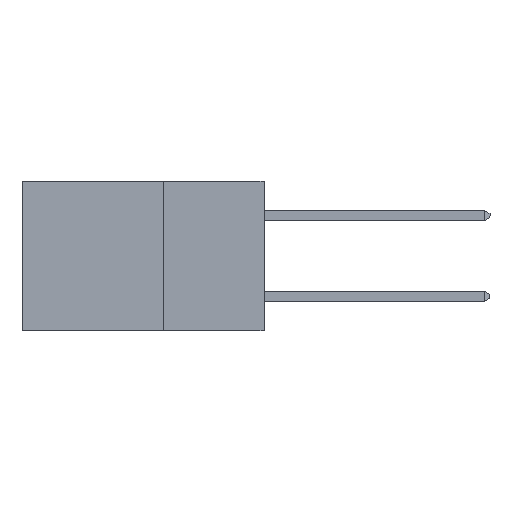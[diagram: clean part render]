
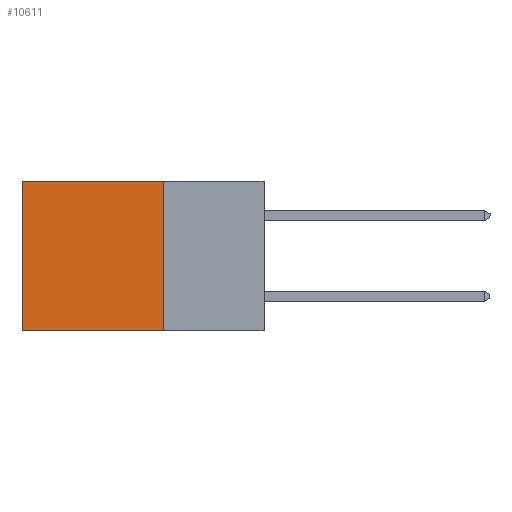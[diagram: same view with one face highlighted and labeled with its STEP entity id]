
A CAD part, left-side view. The second image highlights one B-rep face of the part: STEP entity #10611.
In plain terms, the highlighted planar face has unit normal (-1, 0, 0).
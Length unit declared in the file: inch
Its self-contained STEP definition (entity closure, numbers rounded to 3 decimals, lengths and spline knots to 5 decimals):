
#682 = ORIENTED_EDGE ( 'NONE', *, *, #5136, .F. ) ;
#966 = DIRECTION ( 'NONE',  ( 0., 1., 0. ) ) ;
#1851 = VERTEX_POINT ( 'NONE', #8330 ) ;
#2114 = LINE ( 'NONE', #11177, #6764 ) ;
#2707 = ORIENTED_EDGE ( 'NONE', *, *, #10987, .F. ) ;
#3085 = CARTESIAN_POINT ( 'NONE',  ( 0.298, 0.25, 0. ) ) ;
#3201 = VERTEX_POINT ( 'NONE', #9493 ) ;
#3386 = DIRECTION ( 'NONE',  ( 1., 0., 0. ) ) ;
#3942 = VECTOR ( 'NONE', #6633, 39.37008 ) ;
#4386 = EDGE_LOOP ( 'NONE', ( #4885, #682, #2707, #10275 ) ) ;
#4885 = ORIENTED_EDGE ( 'NONE', *, *, #10183, .T. ) ;
#5136 = EDGE_CURVE ( 'NONE', #7282, #1851, #2114, .T. ) ;
#5416 = CARTESIAN_POINT ( 'NONE',  ( 0.298, 0.6, 0. ) ) ;
#6179 = DIRECTION ( 'NONE',  ( 0., 1., 0. ) ) ;
#6264 = DIRECTION ( 'NONE',  ( 0., 0., -1. ) ) ;
#6286 = LINE ( 'NONE', #3085, #3942 ) ;
#6452 = CARTESIAN_POINT ( 'NONE',  ( 0.298, 0.25, -0.37 ) ) ;
#6633 = DIRECTION ( 'NONE',  ( 0., 0., -1. ) ) ;
#6764 = VECTOR ( 'NONE', #6179, 39.37008 ) ;
#7086 = EDGE_CURVE ( 'NONE', #9172, #3201, #10523, .T. ) ;
#7282 = VERTEX_POINT ( 'NONE', #6452 ) ;
#7370 = VECTOR ( 'NONE', #6264, 39.37008 ) ;
#7472 = LINE ( 'NONE', #5416, #7370 ) ;
#8310 = FACE_OUTER_BOUND ( 'NONE', #4386, .T. ) ;
#8330 = CARTESIAN_POINT ( 'NONE',  ( 0.298, 0.6, -0.37 ) ) ;
#8332 = VECTOR ( 'NONE', #966, 39.37008 ) ;
#8426 = AXIS2_PLACEMENT_3D ( 'NONE', #8607, #3386, #9435 ) ;
#8607 = CARTESIAN_POINT ( 'NONE',  ( 0.298, 0.25, 0. ) ) ;
#8758 = CARTESIAN_POINT ( 'NONE',  ( 0.298, 0.25, 0. ) ) ;
#9141 = CARTESIAN_POINT ( 'NONE',  ( 0.298, 0.25, 0. ) ) ;
#9172 = VERTEX_POINT ( 'NONE', #9141 ) ;
#9435 = DIRECTION ( 'NONE',  ( 0., 0., -1. ) ) ;
#9493 = CARTESIAN_POINT ( 'NONE',  ( 0.298, 0.6, 0. ) ) ;
#10183 = EDGE_CURVE ( 'NONE', #3201, #1851, #7472, .T. ) ;
#10275 = ORIENTED_EDGE ( 'NONE', *, *, #7086, .T. ) ;
#10523 = LINE ( 'NONE', #8758, #8332 ) ;
#10611 = ADVANCED_FACE ( 'NONE', ( #8310 ), #11049, .F. ) ;
#10987 = EDGE_CURVE ( 'NONE', #9172, #7282, #6286, .T. ) ;
#11049 = PLANE ( 'NONE',  #8426 ) ;
#11177 = CARTESIAN_POINT ( 'NONE',  ( 0.298, 0.25, -0.37 ) ) ;
